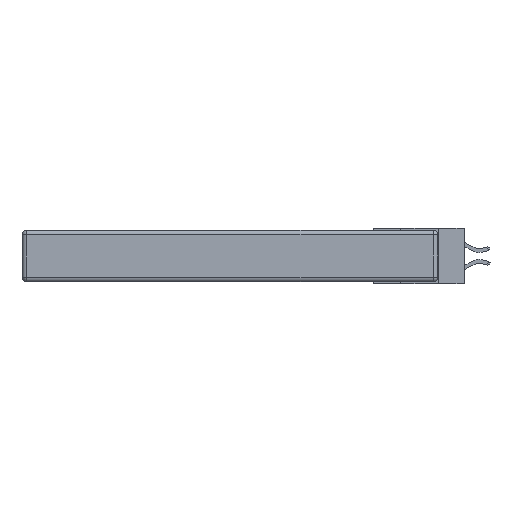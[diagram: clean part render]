
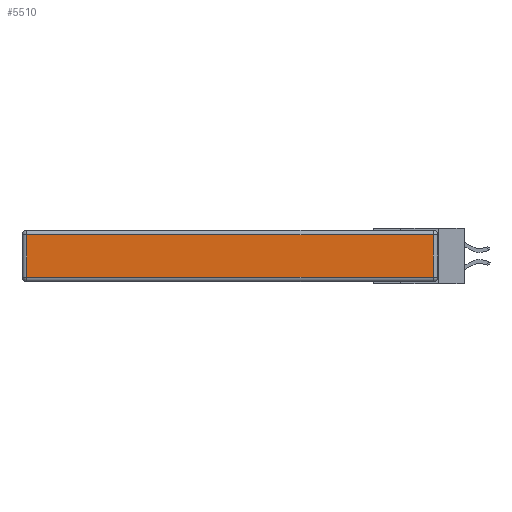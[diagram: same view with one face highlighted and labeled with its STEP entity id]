
A CAD part, left-side view. The second image highlights one B-rep face of the part: STEP entity #5510.
In plain terms, the highlighted planar face has unit normal (-1, 0, 0).
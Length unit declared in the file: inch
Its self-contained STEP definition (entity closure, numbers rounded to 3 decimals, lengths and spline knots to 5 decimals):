
#60 = AXIS2_PLACEMENT_3D ( 'NONE', #16119, #19368, #4025 ) ;
#1778 = ORIENTED_EDGE ( 'NONE', *, *, #8499, .T. ) ;
#2188 = VERTEX_POINT ( 'NONE', #12869 ) ;
#2247 = EDGE_CURVE ( 'NONE', #17503, #7178, #20025, .T. ) ;
#2596 = DIRECTION ( 'NONE',  ( 0., 0., -1. ) ) ;
#4025 = DIRECTION ( 'NONE',  ( 0., 0., 1. ) ) ;
#5440 = DIRECTION ( 'NONE',  ( 0., 1., 0. ) ) ;
#5510 = ADVANCED_FACE ( 'NONE', ( #20635 ), #7383, .T. ) ;
#6060 = EDGE_CURVE ( 'NONE', #7178, #19319, #14996, .T. ) ;
#6352 = VECTOR ( 'NONE', #2596, 39.37008 ) ;
#7178 = VERTEX_POINT ( 'NONE', #17396 ) ;
#7339 = VECTOR ( 'NONE', #8293, 39.37008 ) ;
#7383 = PLANE ( 'NONE',  #60 ) ;
#8293 = DIRECTION ( 'NONE',  ( 0., 0., 1. ) ) ;
#8499 = EDGE_CURVE ( 'NONE', #2188, #17503, #14383, .T. ) ;
#8932 = LINE ( 'NONE', #15096, #7339 ) ;
#10277 = CARTESIAN_POINT ( 'NONE',  ( 0., 2.75, -0.03 ) ) ;
#11068 = CARTESIAN_POINT ( 'NONE',  ( 0., 2.72, -0.343 ) ) ;
#11399 = CARTESIAN_POINT ( 'NONE',  ( 0., 0., -0.313 ) ) ;
#12231 = VECTOR ( 'NONE', #5440, 39.37008 ) ;
#12247 = ORIENTED_EDGE ( 'NONE', *, *, #6060, .T. ) ;
#12869 = CARTESIAN_POINT ( 'NONE',  ( 0., 0.03, -0.03 ) ) ;
#12979 = EDGE_CURVE ( 'NONE', #19319, #2188, #8932, .T. ) ;
#13666 = ORIENTED_EDGE ( 'NONE', *, *, #12979, .T. ) ;
#14383 = LINE ( 'NONE', #10277, #12231 ) ;
#14703 = ORIENTED_EDGE ( 'NONE', *, *, #2247, .T. ) ;
#14996 = LINE ( 'NONE', #11399, #17144 ) ;
#15096 = CARTESIAN_POINT ( 'NONE',  ( 0., 0.03, -0.343 ) ) ;
#16119 = CARTESIAN_POINT ( 'NONE',  ( 0., 0., -0.343 ) ) ;
#17040 = CARTESIAN_POINT ( 'NONE',  ( 0., 0.03, -0.313 ) ) ;
#17144 = VECTOR ( 'NONE', #18083, 39.37008 ) ;
#17396 = CARTESIAN_POINT ( 'NONE',  ( 0., 2.72, -0.313 ) ) ;
#17503 = VERTEX_POINT ( 'NONE', #21159 ) ;
#18083 = DIRECTION ( 'NONE',  ( 0., -1., 0. ) ) ;
#19319 = VERTEX_POINT ( 'NONE', #17040 ) ;
#19368 = DIRECTION ( 'NONE',  ( -1., 0., 0. ) ) ;
#20025 = LINE ( 'NONE', #11068, #6352 ) ;
#20635 = FACE_OUTER_BOUND ( 'NONE', #21164, .T. ) ;
#21159 = CARTESIAN_POINT ( 'NONE',  ( 0., 2.72, -0.03 ) ) ;
#21164 = EDGE_LOOP ( 'NONE', ( #12247, #13666, #1778, #14703 ) ) ;
